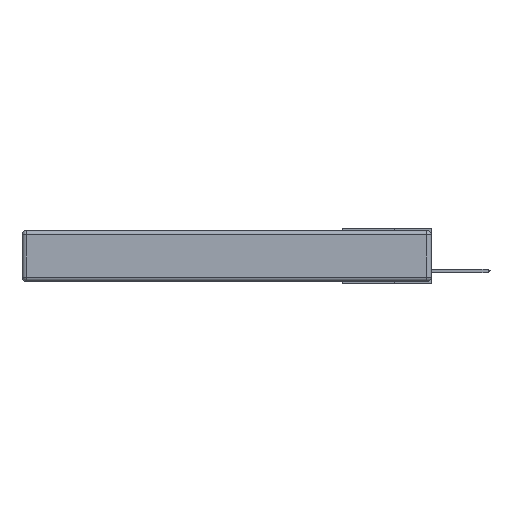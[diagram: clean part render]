
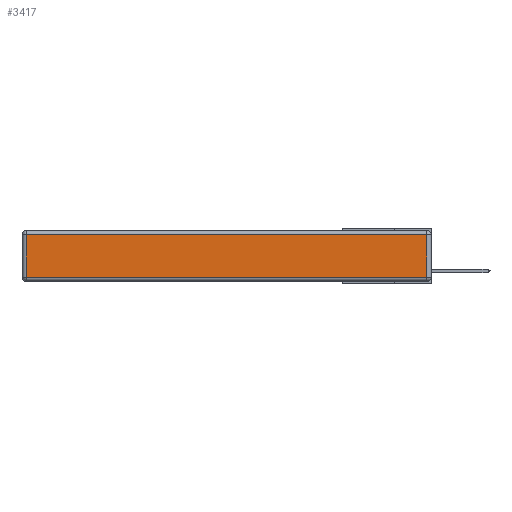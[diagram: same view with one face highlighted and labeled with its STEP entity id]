
A CAD part, left-side view. The second image highlights one B-rep face of the part: STEP entity #3417.
In plain terms, the highlighted planar face has unit normal (-1, 0, 0).
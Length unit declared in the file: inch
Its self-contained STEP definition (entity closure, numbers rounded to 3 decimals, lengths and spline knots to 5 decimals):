
#412 = LINE ( 'NONE', #3912, #12835 ) ;
#548 = PLANE ( 'NONE',  #8355 ) ;
#934 = EDGE_CURVE ( 'NONE', #5589, #14091, #412, .T. ) ;
#1193 = VECTOR ( 'NONE', #9268, 39.37008 ) ;
#1258 = LINE ( 'NONE', #3364, #1811 ) ;
#1811 = VECTOR ( 'NONE', #9174, 39.37008 ) ;
#1921 = EDGE_CURVE ( 'NONE', #5260, #5589, #10767, .T. ) ;
#2668 = ORIENTED_EDGE ( 'NONE', *, *, #3296, .T. ) ;
#3052 = CARTESIAN_POINT ( 'NONE',  ( 0., 0.03, -0.03 ) ) ;
#3296 = EDGE_CURVE ( 'NONE', #9331, #5260, #4757, .T. ) ;
#3364 = CARTESIAN_POINT ( 'NONE',  ( 0., 2.72, -0.343 ) ) ;
#3417 = ADVANCED_FACE ( 'NONE', ( #3628 ), #548, .T. ) ;
#3436 = DIRECTION ( 'NONE',  ( 0., -1., 0. ) ) ;
#3628 = FACE_OUTER_BOUND ( 'NONE', #6225, .T. ) ;
#3912 = CARTESIAN_POINT ( 'NONE',  ( 0., 2.75, -0.03 ) ) ;
#4217 = CARTESIAN_POINT ( 'NONE',  ( 0., 0., -0.343 ) ) ;
#4757 = LINE ( 'NONE', #11792, #15070 ) ;
#5019 = ORIENTED_EDGE ( 'NONE', *, *, #6072, .T. ) ;
#5260 = VERTEX_POINT ( 'NONE', #14349 ) ;
#5589 = VERTEX_POINT ( 'NONE', #3052 ) ;
#6072 = EDGE_CURVE ( 'NONE', #14091, #9331, #1258, .T. ) ;
#6225 = EDGE_LOOP ( 'NONE', ( #2668, #10220, #10946, #5019 ) ) ;
#6716 = CARTESIAN_POINT ( 'NONE',  ( 0., 0.03, -0.343 ) ) ;
#8355 = AXIS2_PLACEMENT_3D ( 'NONE', #4217, #8749, #10051 ) ;
#8749 = DIRECTION ( 'NONE',  ( -1., 0., 0. ) ) ;
#9174 = DIRECTION ( 'NONE',  ( 0., 0., -1. ) ) ;
#9268 = DIRECTION ( 'NONE',  ( 0., 0., 1. ) ) ;
#9331 = VERTEX_POINT ( 'NONE', #10283 ) ;
#9427 = DIRECTION ( 'NONE',  ( 0., 1., 0. ) ) ;
#10051 = DIRECTION ( 'NONE',  ( 0., 0., 1. ) ) ;
#10220 = ORIENTED_EDGE ( 'NONE', *, *, #1921, .T. ) ;
#10283 = CARTESIAN_POINT ( 'NONE',  ( 0., 2.72, -0.313 ) ) ;
#10767 = LINE ( 'NONE', #6716, #1193 ) ;
#10946 = ORIENTED_EDGE ( 'NONE', *, *, #934, .T. ) ;
#11792 = CARTESIAN_POINT ( 'NONE',  ( 0., 0., -0.313 ) ) ;
#12607 = CARTESIAN_POINT ( 'NONE',  ( 0., 2.72, -0.03 ) ) ;
#12835 = VECTOR ( 'NONE', #9427, 39.37008 ) ;
#14091 = VERTEX_POINT ( 'NONE', #12607 ) ;
#14349 = CARTESIAN_POINT ( 'NONE',  ( 0., 0.03, -0.313 ) ) ;
#15070 = VECTOR ( 'NONE', #3436, 39.37008 ) ;
